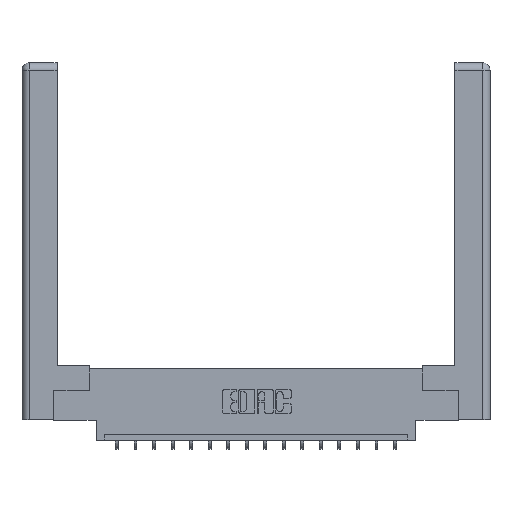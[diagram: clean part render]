
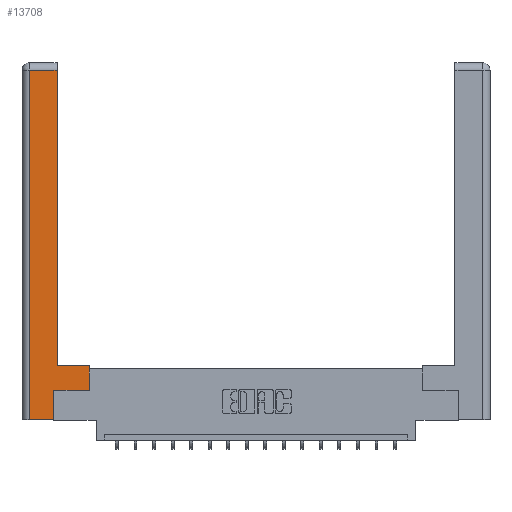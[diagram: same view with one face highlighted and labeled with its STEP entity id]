
A CAD part, top view. The second image highlights one B-rep face of the part: STEP entity #13708.
In plain terms, the highlighted planar face has unit normal (0, 0, 1).
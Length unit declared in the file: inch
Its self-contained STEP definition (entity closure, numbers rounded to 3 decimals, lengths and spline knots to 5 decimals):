
#388 = DIRECTION ( 'NONE',  ( 0., 0., -1. ) ) ;
#664 = LINE ( 'NONE', #14871, #8529 ) ;
#842 = VERTEX_POINT ( 'NONE', #14129 ) ;
#1095 = CARTESIAN_POINT ( 'NONE',  ( 0.565, 0.45, 0. ) ) ;
#1465 = DIRECTION ( 'NONE',  ( 1., 0., 0. ) ) ;
#2123 = CARTESIAN_POINT ( 'NONE',  ( 0.295, 2.94, 0. ) ) ;
#2241 = VERTEX_POINT ( 'NONE', #6628 ) ;
#2317 = VECTOR ( 'NONE', #10443, 39.37008 ) ;
#2770 = LINE ( 'NONE', #16514, #17140 ) ;
#3174 = CARTESIAN_POINT ( 'NONE',  ( 0.565, 0.245, 0. ) ) ;
#3819 = EDGE_CURVE ( 'NONE', #842, #5708, #9800, .T. ) ;
#4180 = DIRECTION ( 'NONE',  ( 0., -1., 0. ) ) ;
#4222 = EDGE_CURVE ( 'NONE', #5708, #8400, #9129, .T. ) ;
#4345 = VECTOR ( 'NONE', #1465, 39.37008 ) ;
#4752 = ORIENTED_EDGE ( 'NONE', *, *, #17674, .T. ) ;
#4867 = CARTESIAN_POINT ( 'NONE',  ( 0., 0., 0. ) ) ;
#4944 = DIRECTION ( 'NONE',  ( -1., 0., 0. ) ) ;
#5294 = ORIENTED_EDGE ( 'NONE', *, *, #17895, .T. ) ;
#5708 = VERTEX_POINT ( 'NONE', #16085 ) ;
#5809 = ORIENTED_EDGE ( 'NONE', *, *, #8538, .T. ) ;
#6019 = VECTOR ( 'NONE', #13921, 39.37008 ) ;
#6076 = VECTOR ( 'NONE', #15647, 39.37008 ) ;
#6168 = AXIS2_PLACEMENT_3D ( 'NONE', #4867, #388, #10120 ) ;
#6628 = CARTESIAN_POINT ( 'NONE',  ( 0.0615, 2.94, 0. ) ) ;
#7034 = VECTOR ( 'NONE', #4180, 39.37008 ) ;
#7200 = EDGE_LOOP ( 'NONE', ( #13492, #4752, #8602, #13573, #12027, #17613, #5294, #5809 ) ) ;
#7330 = CARTESIAN_POINT ( 'NONE',  ( 0.265, 0.245, 0. ) ) ;
#7789 = CARTESIAN_POINT ( 'NONE',  ( 0.295, 0.45, 0. ) ) ;
#8193 = LINE ( 'NONE', #15245, #6019 ) ;
#8234 = CARTESIAN_POINT ( 'NONE',  ( 0.295, 0.45, 0. ) ) ;
#8400 = VERTEX_POINT ( 'NONE', #3174 ) ;
#8529 = VECTOR ( 'NONE', #14811, 39.37008 ) ;
#8538 = EDGE_CURVE ( 'NONE', #15578, #14114, #16301, .T. ) ;
#8602 = ORIENTED_EDGE ( 'NONE', *, *, #14004, .T. ) ;
#9076 = LINE ( 'NONE', #16090, #2317 ) ;
#9129 = LINE ( 'NONE', #11308, #4345 ) ;
#9800 = LINE ( 'NONE', #7330, #6076 ) ;
#10120 = DIRECTION ( 'NONE',  ( -1., 0., 0. ) ) ;
#10443 = DIRECTION ( 'NONE',  ( -1., 0., 0. ) ) ;
#10717 = CARTESIAN_POINT ( 'NONE',  ( 0.0615, 0., 0. ) ) ;
#11308 = CARTESIAN_POINT ( 'NONE',  ( 0.565, 0.245, 0. ) ) ;
#11396 = LINE ( 'NONE', #16920, #7034 ) ;
#11866 = VERTEX_POINT ( 'NONE', #10717 ) ;
#12027 = ORIENTED_EDGE ( 'NONE', *, *, #3819, .T. ) ;
#12947 = FACE_OUTER_BOUND ( 'NONE', #7200, .T. ) ;
#13492 = ORIENTED_EDGE ( 'NONE', *, *, #17814, .T. ) ;
#13573 = ORIENTED_EDGE ( 'NONE', *, *, #14760, .T. ) ;
#13708 = ADVANCED_FACE ( 'NONE', ( #12947 ), #16931, .F. ) ;
#13921 = DIRECTION ( 'NONE',  ( 0., 1., 0. ) ) ;
#14004 = EDGE_CURVE ( 'NONE', #2241, #11866, #11396, .T. ) ;
#14114 = VERTEX_POINT ( 'NONE', #8234 ) ;
#14129 = CARTESIAN_POINT ( 'NONE',  ( 0.265, 0., 0. ) ) ;
#14760 = EDGE_CURVE ( 'NONE', #11866, #842, #664, .T. ) ;
#14811 = DIRECTION ( 'NONE',  ( 1., 0., 0. ) ) ;
#14871 = CARTESIAN_POINT ( 'NONE',  ( 0.265, 0., 0. ) ) ;
#15245 = CARTESIAN_POINT ( 'NONE',  ( 0.565, 0.45, 0. ) ) ;
#15578 = VERTEX_POINT ( 'NONE', #1095 ) ;
#15647 = DIRECTION ( 'NONE',  ( 0., 1., 0. ) ) ;
#16085 = CARTESIAN_POINT ( 'NONE',  ( 0.265, 0.245, 0. ) ) ;
#16090 = CARTESIAN_POINT ( 'NONE',  ( 0.0615, 2.94, 0. ) ) ;
#16301 = LINE ( 'NONE', #7789, #17167 ) ;
#16514 = CARTESIAN_POINT ( 'NONE',  ( 0.295, 3., 0. ) ) ;
#16920 = CARTESIAN_POINT ( 'NONE',  ( 0.0615, 0., 0. ) ) ;
#16931 = PLANE ( 'NONE',  #6168 ) ;
#17140 = VECTOR ( 'NONE', #17600, 39.37008 ) ;
#17167 = VECTOR ( 'NONE', #4944, 39.37008 ) ;
#17556 = VERTEX_POINT ( 'NONE', #2123 ) ;
#17600 = DIRECTION ( 'NONE',  ( 0., 1., 0. ) ) ;
#17613 = ORIENTED_EDGE ( 'NONE', *, *, #4222, .T. ) ;
#17674 = EDGE_CURVE ( 'NONE', #17556, #2241, #9076, .T. ) ;
#17814 = EDGE_CURVE ( 'NONE', #14114, #17556, #2770, .T. ) ;
#17895 = EDGE_CURVE ( 'NONE', #8400, #15578, #8193, .T. ) ;
